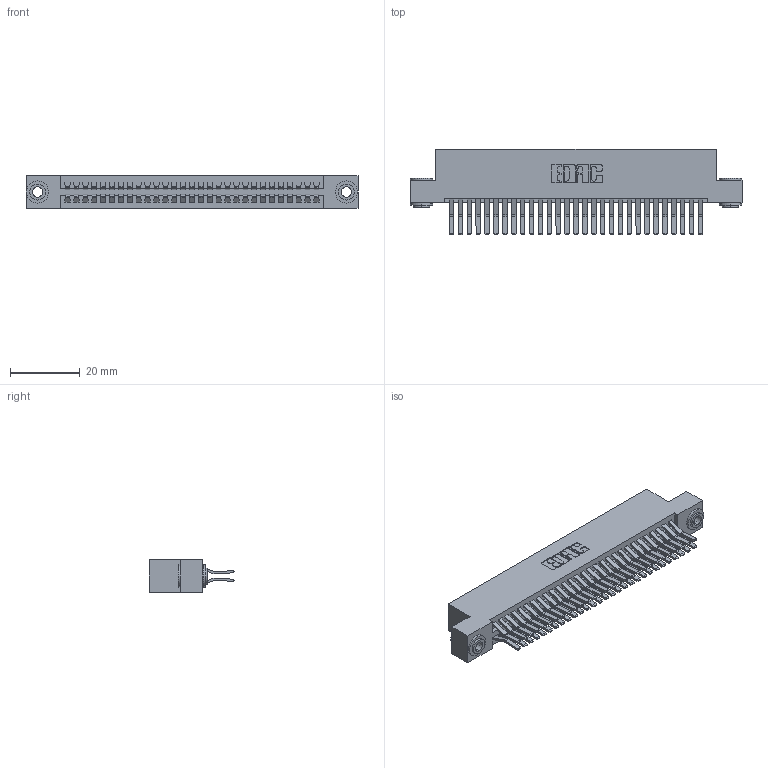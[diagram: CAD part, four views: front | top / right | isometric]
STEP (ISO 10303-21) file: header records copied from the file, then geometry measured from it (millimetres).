
FILE_DESCRIPTION (( 'STEP AP203' ), '1' );
FILE_NAME ('345-058-560-203.STEP', '2018-09-26T18:43:21', ( '' ), ( '' ), 'SwSTEP 2.0', 'SolidWorks 2016', '' );
FILE_SCHEMA (( 'CONFIG_CONTROL_DESIGN' ));
Length unit declared in the file: inch
Products named in the file (4): 345-292-001_560 Tail; 345 Part_Flush Mounting Lugs - 0.156 Dia-TH; 345-058-560-203; 345-250-002_345-250-002-102
Assembly tree (61 placements, depth 2):
  345-058-560-203
    345 Part_Flush Mounting Lugs - 0.156 Dia-TH
    345-292-001_560 Tail  x58
    345-250-002_345-250-002-102  x2
Bounding box: 94.87 x 24.45 x 9.4 mm (x, y, z)
Volume: 9494.6 mm3; surface area: 14965.4 mm2
Topology: 61 solids, 61 shells, 3180 faces, 9407 edges, 6190 vertices
Faces by surface type: plane 2004, cylinder 1168, cone 8
Entity records: 25242 total; most frequent: CARTESIAN_POINT 4219, ORIENTED_EDGE 4146, DIRECTION 3771, EDGE_CURVE 2073, VECTOR 1797, LINE 1797, VERTEX_POINT 1378, AXIS2_PLACEMENT_3D 987
